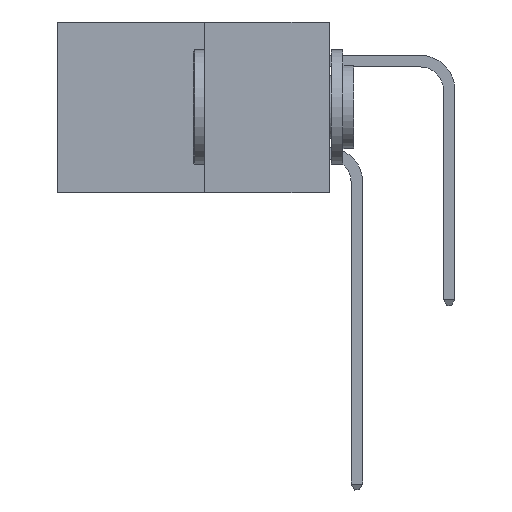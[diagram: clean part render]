
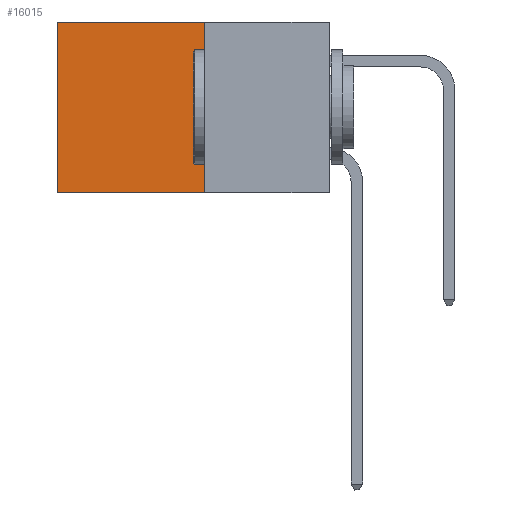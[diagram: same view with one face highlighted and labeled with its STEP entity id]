
A CAD part, left-side view. The second image highlights one B-rep face of the part: STEP entity #16015.
In plain terms, the highlighted planar face has unit normal (-1, 0, 0).
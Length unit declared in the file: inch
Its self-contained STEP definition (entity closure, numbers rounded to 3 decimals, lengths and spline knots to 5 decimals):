
#1080 = VERTEX_POINT ( 'NONE', #27113 ) ;
#1991 = ORIENTED_EDGE ( 'NONE', *, *, #10474, .T. ) ;
#3541 = ORIENTED_EDGE ( 'NONE', *, *, #5356, .F. ) ;
#5356 = EDGE_CURVE ( 'NONE', #1080, #11674, #11623, .T. ) ;
#5453 = CARTESIAN_POINT ( 'NONE',  ( 0.277, 0.59, -0.37 ) ) ;
#6150 = EDGE_LOOP ( 'NONE', ( #10936, #3541, #28624, #1991 ) ) ;
#7989 = LINE ( 'NONE', #5453, #19348 ) ;
#9334 = CARTESIAN_POINT ( 'NONE',  ( 0.277, 0.27, -0.37 ) ) ;
#9641 = EDGE_CURVE ( 'NONE', #13075, #1080, #15329, .T. ) ;
#9742 = DIRECTION ( 'NONE',  ( 0., 0., -1. ) ) ;
#10474 = EDGE_CURVE ( 'NONE', #13075, #16186, #14230, .T. ) ;
#10936 = ORIENTED_EDGE ( 'NONE', *, *, #18164, .T. ) ;
#11623 = LINE ( 'NONE', #26445, #21557 ) ;
#11637 = DIRECTION ( 'NONE',  ( 0., 0., -1. ) ) ;
#11674 = VERTEX_POINT ( 'NONE', #23605 ) ;
#11782 = CARTESIAN_POINT ( 'NONE',  ( 0.277, 0.27, 0. ) ) ;
#13075 = VERTEX_POINT ( 'NONE', #11782 ) ;
#14230 = LINE ( 'NONE', #28500, #20231 ) ;
#14336 = CARTESIAN_POINT ( 'NONE',  ( 0.277, 0.27, -0.37 ) ) ;
#15104 = DIRECTION ( 'NONE',  ( 0., 1., 0. ) ) ;
#15329 = LINE ( 'NONE', #14336, #27937 ) ;
#16015 = ADVANCED_FACE ( 'NONE', ( #28654 ), #22920, .F. ) ;
#16186 = VERTEX_POINT ( 'NONE', #16699 ) ;
#16699 = CARTESIAN_POINT ( 'NONE',  ( 0.277, 0.59, 0. ) ) ;
#16939 = AXIS2_PLACEMENT_3D ( 'NONE', #9334, #25138, #11637 ) ;
#18164 = EDGE_CURVE ( 'NONE', #16186, #11674, #7989, .T. ) ;
#19059 = DIRECTION ( 'NONE',  ( 0., 0., -1. ) ) ;
#19348 = VECTOR ( 'NONE', #19059, 39.37008 ) ;
#20231 = VECTOR ( 'NONE', #15104, 39.37008 ) ;
#21557 = VECTOR ( 'NONE', #25921, 39.37008 ) ;
#22920 = PLANE ( 'NONE',  #16939 ) ;
#23605 = CARTESIAN_POINT ( 'NONE',  ( 0.277, 0.59, -0.37 ) ) ;
#25138 = DIRECTION ( 'NONE',  ( 1., 0., 0. ) ) ;
#25921 = DIRECTION ( 'NONE',  ( 0., 1., 0. ) ) ;
#26445 = CARTESIAN_POINT ( 'NONE',  ( 0.277, 0.27, -0.37 ) ) ;
#27113 = CARTESIAN_POINT ( 'NONE',  ( 0.277, 0.27, -0.37 ) ) ;
#27937 = VECTOR ( 'NONE', #9742, 39.37008 ) ;
#28500 = CARTESIAN_POINT ( 'NONE',  ( 0.277, 0.27, 0. ) ) ;
#28624 = ORIENTED_EDGE ( 'NONE', *, *, #9641, .F. ) ;
#28654 = FACE_OUTER_BOUND ( 'NONE', #6150, .T. ) ;
